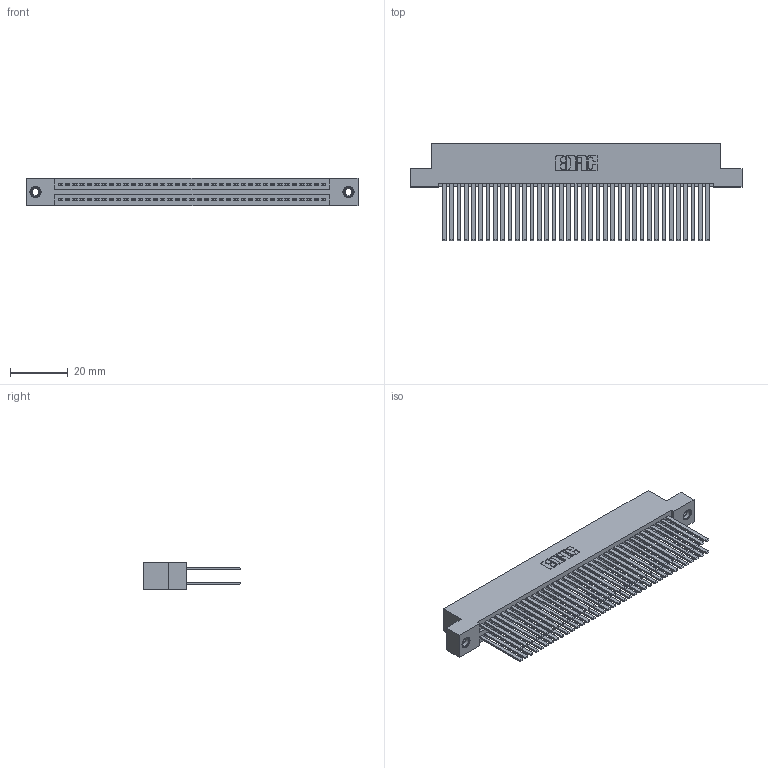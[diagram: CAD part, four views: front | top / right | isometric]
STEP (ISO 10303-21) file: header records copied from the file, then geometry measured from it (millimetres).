
FILE_DESCRIPTION (( 'STEP AP203' ), '1' );
FILE_NAME ('395-074-544-208.STEP', '2018-11-27T19:14:12', ( '' ), ( '' ), 'SwSTEP 2.0', 'SolidWorks 2016', '' );
FILE_SCHEMA (( 'CONFIG_CONTROL_DESIGN' ));
Length unit declared in the file: inch
Products named in the file (4): 395-074-544-208; 345-292-001_345-293-144; 345-250-001_345-250-003-102; 345 Part_Flush Mounting Lugs - 0.156 Dia-TI
Assembly tree (77 placements, depth 2):
  395-074-544-208
    345 Part_Flush Mounting Lugs - 0.156 Dia-TI
    345-292-001_345-293-144  x74
    345-250-001_345-250-003-102  x2
Bounding box: 115.19 x 33.96 x 9.4 mm (x, y, z)
Volume: 12174 mm3; surface area: 20952.2 mm2
Topology: 77 solids, 77 shells, 3442 faces, 10171 edges, 6674 vertices
Faces by surface type: plane 2258, cylinder 1168, cone 12, torus 4
Entity records: 30706 total; most frequent: CARTESIAN_POINT 5131, ORIENTED_EDGE 5058, DIRECTION 4555, EDGE_CURVE 2529, LINE 2233, VECTOR 2233, VERTEX_POINT 1680, AXIS2_PLACEMENT_3D 1161
